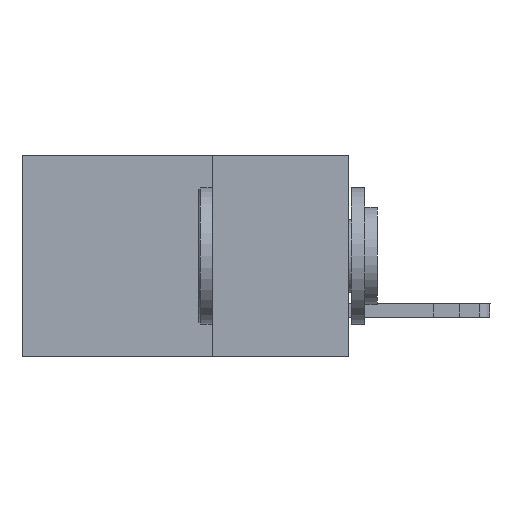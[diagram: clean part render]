
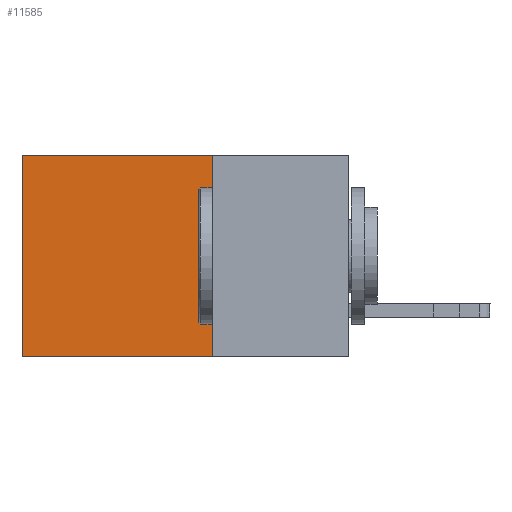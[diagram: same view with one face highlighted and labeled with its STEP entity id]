
A CAD part, left-side view. The second image highlights one B-rep face of the part: STEP entity #11585.
In plain terms, the highlighted planar face has unit normal (-1, 0, 0).
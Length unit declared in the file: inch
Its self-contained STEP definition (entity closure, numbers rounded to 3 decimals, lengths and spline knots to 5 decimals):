
#81 = DIRECTION ( 'NONE',  ( 0., 0., -1. ) ) ;
#569 = CARTESIAN_POINT ( 'NONE',  ( 0.298, 0.6, 0. ) ) ;
#952 = VERTEX_POINT ( 'NONE', #13319 ) ;
#1275 = VERTEX_POINT ( 'NONE', #7411 ) ;
#2140 = VECTOR ( 'NONE', #5846, 39.37008 ) ;
#2169 = DIRECTION ( 'NONE',  ( 0., 1., 0. ) ) ;
#2488 = EDGE_CURVE ( 'NONE', #952, #12813, #7765, .T. ) ;
#2868 = EDGE_CURVE ( 'NONE', #1275, #12813, #13631, .T. ) ;
#3198 = DIRECTION ( 'NONE',  ( 0., 0., -1. ) ) ;
#3301 = CARTESIAN_POINT ( 'NONE',  ( 0.298, 0.6, -0.37 ) ) ;
#4483 = LINE ( 'NONE', #15034, #15844 ) ;
#5071 = ORIENTED_EDGE ( 'NONE', *, *, #13326, .F. ) ;
#5761 = VERTEX_POINT ( 'NONE', #13620 ) ;
#5846 = DIRECTION ( 'NONE',  ( 0., 0., -1. ) ) ;
#6302 = DIRECTION ( 'NONE',  ( 0., 1., 0. ) ) ;
#7109 = VECTOR ( 'NONE', #6302, 39.37008 ) ;
#7411 = CARTESIAN_POINT ( 'NONE',  ( 0.298, 0.6, 0. ) ) ;
#7765 = LINE ( 'NONE', #12876, #7109 ) ;
#8182 = EDGE_LOOP ( 'NONE', ( #10588, #12147, #5071, #10459 ) ) ;
#8219 = FACE_OUTER_BOUND ( 'NONE', #8182, .T. ) ;
#10459 = ORIENTED_EDGE ( 'NONE', *, *, #16005, .T. ) ;
#10588 = ORIENTED_EDGE ( 'NONE', *, *, #2868, .T. ) ;
#11585 = ADVANCED_FACE ( 'NONE', ( #8219 ), #13484, .F. ) ;
#11938 = DIRECTION ( 'NONE',  ( 1., 0., 0. ) ) ;
#12147 = ORIENTED_EDGE ( 'NONE', *, *, #2488, .F. ) ;
#12568 = VECTOR ( 'NONE', #2169, 39.37008 ) ;
#12813 = VERTEX_POINT ( 'NONE', #3301 ) ;
#12876 = CARTESIAN_POINT ( 'NONE',  ( 0.298, 0.25, -0.37 ) ) ;
#13319 = CARTESIAN_POINT ( 'NONE',  ( 0.298, 0.25, -0.37 ) ) ;
#13326 = EDGE_CURVE ( 'NONE', #5761, #952, #4483, .T. ) ;
#13484 = PLANE ( 'NONE',  #14425 ) ;
#13620 = CARTESIAN_POINT ( 'NONE',  ( 0.298, 0.25, 0. ) ) ;
#13631 = LINE ( 'NONE', #569, #2140 ) ;
#14006 = CARTESIAN_POINT ( 'NONE',  ( 0.298, 0.25, 0. ) ) ;
#14425 = AXIS2_PLACEMENT_3D ( 'NONE', #16152, #11938, #81 ) ;
#15034 = CARTESIAN_POINT ( 'NONE',  ( 0.298, 0.25, 0. ) ) ;
#15844 = VECTOR ( 'NONE', #3198, 39.37008 ) ;
#16005 = EDGE_CURVE ( 'NONE', #5761, #1275, #16764, .T. ) ;
#16152 = CARTESIAN_POINT ( 'NONE',  ( 0.298, 0.25, 0. ) ) ;
#16764 = LINE ( 'NONE', #14006, #12568 ) ;
